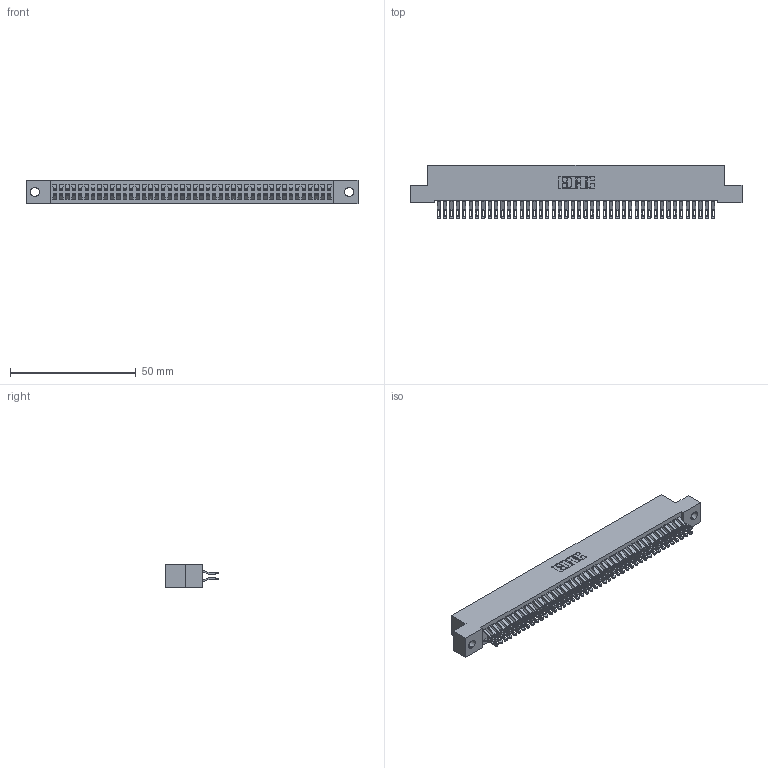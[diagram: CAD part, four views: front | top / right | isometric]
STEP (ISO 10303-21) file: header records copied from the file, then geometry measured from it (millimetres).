
FILE_DESCRIPTION (( 'STEP AP203' ), '1' );
FILE_NAME ('392-088-555-202.STEP', '2019-10-09T16:57:23', ( '' ), ( '' ), 'SwSTEP 2.0', 'SolidWorks 2016', '' );
FILE_SCHEMA (( 'CONFIG_CONTROL_DESIGN' ));
Length unit declared in the file: inch
Products named in the file (3): 342 Part_.128 Slot; 345-292-001_555 Tail; 392-088-555-202
Assembly tree (89 placements, depth 2):
  392-088-555-202
    342 Part_.128 Slot
    345-292-001_555 Tail  x88
Bounding box: 132.08 x 21.47 x 9.4 mm (x, y, z)
Volume: 12069.2 mm3; surface area: 20305.9 mm2
Topology: 89 solids, 89 shells, 5218 faces, 16415 edges, 10942 vertices
Faces by surface type: plane 3062, cylinder 2156
Entity records: 28377 total; most frequent: CARTESIAN_POINT 4736, ORIENTED_EDGE 4642, DIRECTION 4013, EDGE_CURVE 2321, VECTOR 2173, LINE 2173, VERTEX_POINT 1546, AXIS2_PLACEMENT_3D 920
